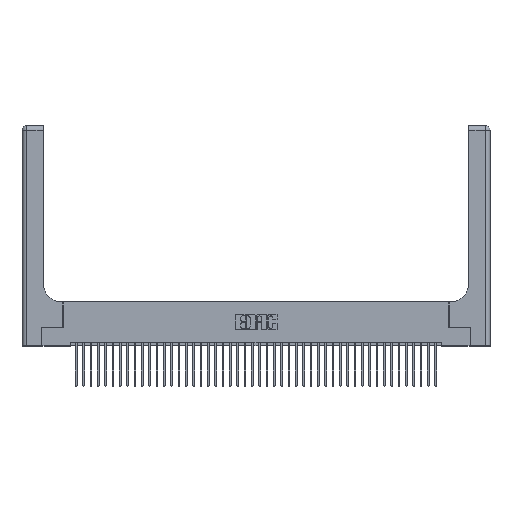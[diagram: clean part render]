
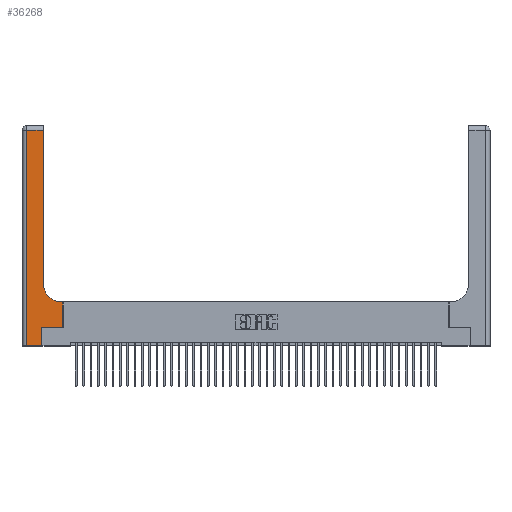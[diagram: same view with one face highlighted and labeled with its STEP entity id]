
A CAD part, top view. The second image highlights one B-rep face of the part: STEP entity #36268.
In plain terms, the highlighted planar face has unit normal (0, 0, 1).
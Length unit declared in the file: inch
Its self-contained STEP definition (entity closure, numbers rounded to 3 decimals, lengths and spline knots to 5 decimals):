
#248 = AXIS2_PLACEMENT_3D ( 'NONE', #14050, #3811, #3952 ) ;
#301 = VERTEX_POINT ( 'NONE', #3731 ) ;
#761 = CARTESIAN_POINT ( 'NONE',  ( 0.269, 0., 0.37 ) ) ;
#1805 = CARTESIAN_POINT ( 'NONE',  ( 0., 2.94, 0.37 ) ) ;
#1968 = ORIENTED_EDGE ( 'NONE', *, *, #25272, .T. ) ;
#2724 = DIRECTION ( 'NONE',  ( 0., -1., 0. ) ) ;
#3731 = CARTESIAN_POINT ( 'NONE',  ( 0.269, 0., 0.37 ) ) ;
#3765 = ORIENTED_EDGE ( 'NONE', *, *, #4149, .T. ) ;
#3811 = DIRECTION ( 'NONE',  ( 0., 0., -1. ) ) ;
#3952 = DIRECTION ( 'NONE',  ( 1., 0., 0. ) ) ;
#4149 = EDGE_CURVE ( 'NONE', #8414, #4753, #10354, .T. ) ;
#4753 = VERTEX_POINT ( 'NONE', #38447 ) ;
#5800 = CARTESIAN_POINT ( 'NONE',  ( 0.269, 0.25, 0.37 ) ) ;
#6524 = VERTEX_POINT ( 'NONE', #37170 ) ;
#6765 = CARTESIAN_POINT ( 'NONE',  ( 0.2915, 0.85, 0.37 ) ) ;
#6792 = EDGE_LOOP ( 'NONE', ( #36798, #6805, #29411, #30906, #35454, #33272, #3765, #1968, #38642 ) ) ;
#6805 = ORIENTED_EDGE ( 'NONE', *, *, #16983, .T. ) ;
#7265 = DIRECTION ( 'NONE',  ( 1., 0., 0. ) ) ;
#8414 = VERTEX_POINT ( 'NONE', #34500 ) ;
#8720 = LINE ( 'NONE', #36116, #20752 ) ;
#10354 = LINE ( 'NONE', #17553, #15051 ) ;
#10603 = VECTOR ( 'NONE', #32907, 39.37008 ) ;
#10605 = VERTEX_POINT ( 'NONE', #42491 ) ;
#10643 = CIRCLE ( 'NONE', #248, 0.25 ) ;
#11598 = VECTOR ( 'NONE', #20677, 39.37008 ) ;
#11652 = LINE ( 'NONE', #42401, #10603 ) ;
#12222 = LINE ( 'NONE', #34555, #20078 ) ;
#12252 = EDGE_CURVE ( 'NONE', #301, #31665, #28582, .T. ) ;
#12660 = LINE ( 'NONE', #13549, #11598 ) ;
#13549 = CARTESIAN_POINT ( 'NONE',  ( 0.269, 0.25, 0.37 ) ) ;
#13953 = VERTEX_POINT ( 'NONE', #16912 ) ;
#14050 = CARTESIAN_POINT ( 'NONE',  ( 0.5415, 0.85, 0.37 ) ) ;
#15051 = VECTOR ( 'NONE', #27704, 39.37008 ) ;
#15889 = PLANE ( 'NONE',  #43106 ) ;
#16912 = CARTESIAN_POINT ( 'NONE',  ( 0.2915, 2.94, 0.37 ) ) ;
#16983 = EDGE_CURVE ( 'NONE', #13953, #30365, #35902, .T. ) ;
#17200 = VERTEX_POINT ( 'NONE', #6765 ) ;
#17553 = CARTESIAN_POINT ( 'NONE',  ( 0.5585, 0.25, 0.37 ) ) ;
#17858 = EDGE_CURVE ( 'NONE', #10605, #17200, #10643, .T. ) ;
#18202 = VECTOR ( 'NONE', #7265, 39.37008 ) ;
#18218 = EDGE_CURVE ( 'NONE', #17200, #13953, #11652, .T. ) ;
#19106 = DIRECTION ( 'NONE',  ( -1., 0., 0. ) ) ;
#19263 = CARTESIAN_POINT ( 'NONE',  ( 0., 3., 0.37 ) ) ;
#20078 = VECTOR ( 'NONE', #27675, 39.37008 ) ;
#20677 = DIRECTION ( 'NONE',  ( 1., 0., 0. ) ) ;
#20752 = VECTOR ( 'NONE', #2724, 39.37008 ) ;
#22650 = DIRECTION ( 'NONE',  ( 0., 0., -1. ) ) ;
#24902 = VECTOR ( 'NONE', #25560, 39.37008 ) ;
#25272 = EDGE_CURVE ( 'NONE', #4753, #10605, #12222, .T. ) ;
#25560 = DIRECTION ( 'NONE',  ( -1., 0., 0. ) ) ;
#27145 = LINE ( 'NONE', #34099, #18202 ) ;
#27675 = DIRECTION ( 'NONE',  ( -1., 0., 0. ) ) ;
#27704 = DIRECTION ( 'NONE',  ( 0., 1., 0. ) ) ;
#28582 = LINE ( 'NONE', #761, #39494 ) ;
#28929 = EDGE_CURVE ( 'NONE', #31665, #8414, #12660, .T. ) ;
#29411 = ORIENTED_EDGE ( 'NONE', *, *, #36271, .T. ) ;
#30365 = VERTEX_POINT ( 'NONE', #41751 ) ;
#30906 = ORIENTED_EDGE ( 'NONE', *, *, #35813, .T. ) ;
#31665 = VERTEX_POINT ( 'NONE', #5800 ) ;
#32047 = DIRECTION ( 'NONE',  ( 0., 1., 0. ) ) ;
#32328 = FACE_OUTER_BOUND ( 'NONE', #6792, .T. ) ;
#32907 = DIRECTION ( 'NONE',  ( 0., 1., 0. ) ) ;
#33272 = ORIENTED_EDGE ( 'NONE', *, *, #28929, .T. ) ;
#34099 = CARTESIAN_POINT ( 'NONE',  ( 0., 0., 0.37 ) ) ;
#34500 = CARTESIAN_POINT ( 'NONE',  ( 0.5585, 0.25, 0.37 ) ) ;
#34555 = CARTESIAN_POINT ( 'NONE',  ( 0.2915, 0.6, 0.37 ) ) ;
#35454 = ORIENTED_EDGE ( 'NONE', *, *, #12252, .T. ) ;
#35813 = EDGE_CURVE ( 'NONE', #6524, #301, #27145, .T. ) ;
#35902 = LINE ( 'NONE', #1805, #24902 ) ;
#36116 = CARTESIAN_POINT ( 'NONE',  ( 0.06, 3., 0.37 ) ) ;
#36268 = ADVANCED_FACE ( 'NONE', ( #32328 ), #15889, .F. ) ;
#36271 = EDGE_CURVE ( 'NONE', #30365, #6524, #8720, .T. ) ;
#36798 = ORIENTED_EDGE ( 'NONE', *, *, #18218, .T. ) ;
#37170 = CARTESIAN_POINT ( 'NONE',  ( 0.06, 0., 0.37 ) ) ;
#38447 = CARTESIAN_POINT ( 'NONE',  ( 0.5585, 0.6, 0.37 ) ) ;
#38642 = ORIENTED_EDGE ( 'NONE', *, *, #17858, .T. ) ;
#39494 = VECTOR ( 'NONE', #32047, 39.37008 ) ;
#41751 = CARTESIAN_POINT ( 'NONE',  ( 0.06, 2.94, 0.37 ) ) ;
#42401 = CARTESIAN_POINT ( 'NONE',  ( 0.2915, 3., 0.37 ) ) ;
#42491 = CARTESIAN_POINT ( 'NONE',  ( 0.5415, 0.6, 0.37 ) ) ;
#43106 = AXIS2_PLACEMENT_3D ( 'NONE', #19263, #22650, #19106 ) ;
